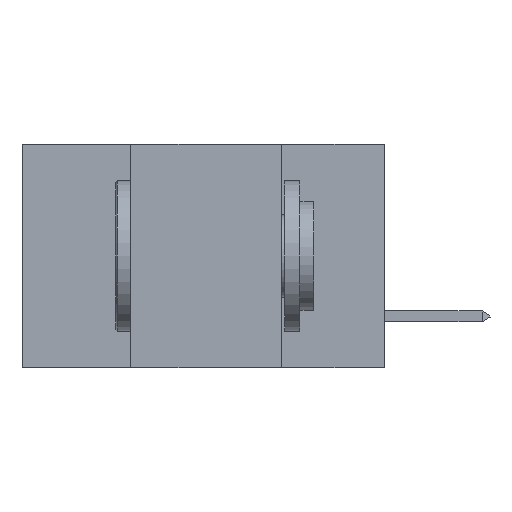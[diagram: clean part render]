
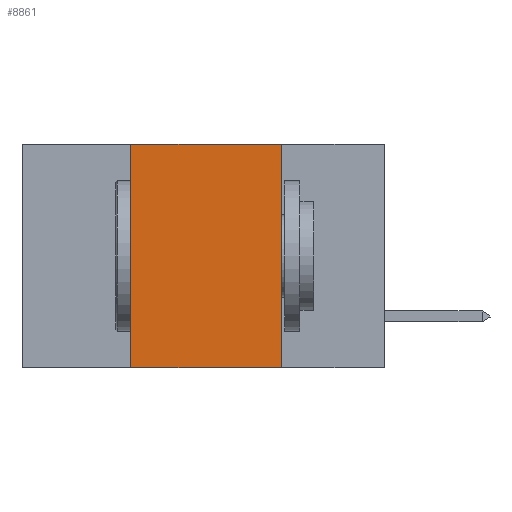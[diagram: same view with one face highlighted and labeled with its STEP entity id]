
A CAD part, left-side view. The second image highlights one B-rep face of the part: STEP entity #8861.
In plain terms, the highlighted planar face has unit normal (-1, 0, 0).
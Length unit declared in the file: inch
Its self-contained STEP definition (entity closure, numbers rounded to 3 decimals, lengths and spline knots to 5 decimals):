
#588 = DIRECTION ( 'NONE',  ( 0., 0., 1. ) ) ;
#2801 = EDGE_CURVE ( 'NONE', #14632, #22177, #13145, .T. ) ;
#4251 = CARTESIAN_POINT ( 'NONE',  ( 0., 0.6, 0. ) ) ;
#4412 = ORIENTED_EDGE ( 'NONE', *, *, #13193, .F. ) ;
#5415 = EDGE_LOOP ( 'NONE', ( #4412, #11961, #12253, #37761 ) ) ;
#7413 = LINE ( 'NONE', #25588, #23086 ) ;
#8861 = ADVANCED_FACE ( 'NONE', ( #24919 ), #11010, .F. ) ;
#8995 = CARTESIAN_POINT ( 'NONE',  ( 0., 0.42, 0. ) ) ;
#9360 = LINE ( 'NONE', #8995, #32793 ) ;
#11010 = PLANE ( 'NONE',  #37976 ) ;
#11149 = DIRECTION ( 'NONE',  ( 0., 0., -1. ) ) ;
#11855 = VERTEX_POINT ( 'NONE', #39866 ) ;
#11961 = ORIENTED_EDGE ( 'NONE', *, *, #2801, .F. ) ;
#12253 = ORIENTED_EDGE ( 'NONE', *, *, #28298, .F. ) ;
#13145 = LINE ( 'NONE', #4251, #37195 ) ;
#13193 = EDGE_CURVE ( 'NONE', #22177, #32256, #23461, .T. ) ;
#14632 = VERTEX_POINT ( 'NONE', #16924 ) ;
#16924 = CARTESIAN_POINT ( 'NONE',  ( 0., 0.42, 0. ) ) ;
#20382 = CARTESIAN_POINT ( 'NONE',  ( 0., 0.17, 0. ) ) ;
#21030 = DIRECTION ( 'NONE',  ( 0., 0., -1. ) ) ;
#21386 = CARTESIAN_POINT ( 'NONE',  ( 0., 0.17, -0.37 ) ) ;
#22177 = VERTEX_POINT ( 'NONE', #20382 ) ;
#23086 = VECTOR ( 'NONE', #31760, 39.37008 ) ;
#23461 = LINE ( 'NONE', #39791, #23919 ) ;
#23919 = VECTOR ( 'NONE', #21030, 39.37008 ) ;
#24919 = FACE_OUTER_BOUND ( 'NONE', #5415, .T. ) ;
#25588 = CARTESIAN_POINT ( 'NONE',  ( 0., 0.6, -0.37 ) ) ;
#26835 = CARTESIAN_POINT ( 'NONE',  ( 0., 0.6, 0. ) ) ;
#28298 = EDGE_CURVE ( 'NONE', #11855, #14632, #9360, .T. ) ;
#29818 = DIRECTION ( 'NONE',  ( 1., 0., 0. ) ) ;
#30003 = EDGE_CURVE ( 'NONE', #11855, #32256, #7413, .T. ) ;
#31760 = DIRECTION ( 'NONE',  ( 0., -1., 0. ) ) ;
#32256 = VERTEX_POINT ( 'NONE', #21386 ) ;
#32363 = DIRECTION ( 'NONE',  ( 0., -1., 0. ) ) ;
#32793 = VECTOR ( 'NONE', #588, 39.37008 ) ;
#37195 = VECTOR ( 'NONE', #32363, 39.37008 ) ;
#37761 = ORIENTED_EDGE ( 'NONE', *, *, #30003, .T. ) ;
#37976 = AXIS2_PLACEMENT_3D ( 'NONE', #26835, #29818, #11149 ) ;
#39791 = CARTESIAN_POINT ( 'NONE',  ( 0., 0.17, 0. ) ) ;
#39866 = CARTESIAN_POINT ( 'NONE',  ( 0., 0.42, -0.37 ) ) ;
